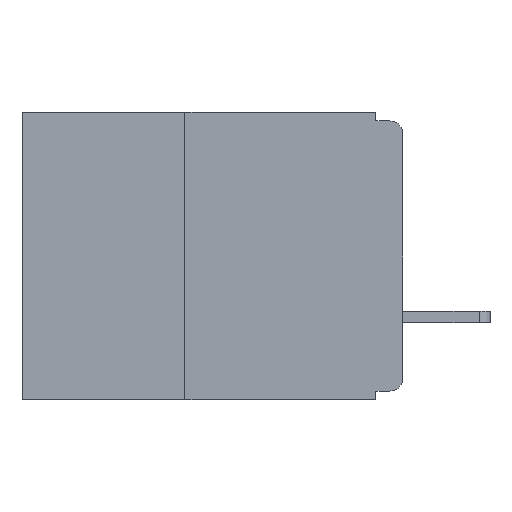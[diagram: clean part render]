
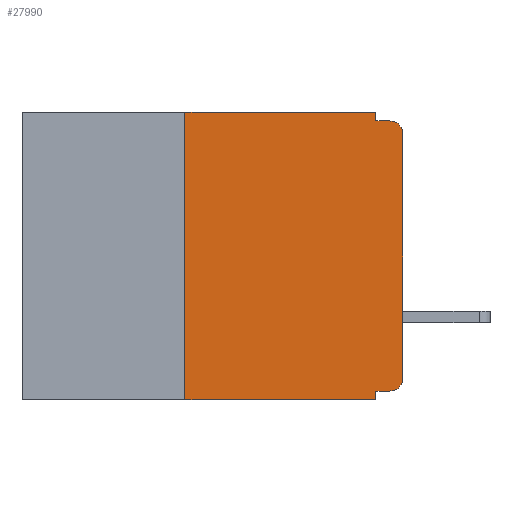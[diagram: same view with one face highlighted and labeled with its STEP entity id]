
A CAD part, left-side view. The second image highlights one B-rep face of the part: STEP entity #27990.
In plain terms, the highlighted planar face has unit normal (-1, 0, 0).
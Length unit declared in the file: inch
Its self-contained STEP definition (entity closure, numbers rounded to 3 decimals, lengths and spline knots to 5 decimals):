
#1207 = DIRECTION ( 'NONE',  ( 0., 0., -1. ) ) ;
#1368 = CARTESIAN_POINT ( 'NONE',  ( 0., 0.015, -0.025 ) ) ;
#1694 = CARTESIAN_POINT ( 'NONE',  ( 0., 0.25, 0. ) ) ;
#2203 = LINE ( 'NONE', #14770, #26049 ) ;
#2496 = ORIENTED_EDGE ( 'NONE', *, *, #6221, .T. ) ;
#2530 = CARTESIAN_POINT ( 'NONE',  ( 0., 0.25, -0.33 ) ) ;
#3075 = DIRECTION ( 'NONE',  ( 0., 1., 0. ) ) ;
#3128 = VERTEX_POINT ( 'NONE', #2530 ) ;
#3298 = VECTOR ( 'NONE', #1207, 39.37008 ) ;
#3785 = DIRECTION ( 'NONE',  ( 0., 0., -1. ) ) ;
#4004 = VERTEX_POINT ( 'NONE', #5722 ) ;
#4083 = CARTESIAN_POINT ( 'NONE',  ( 0., 0.031, 0. ) ) ;
#4739 = CIRCLE ( 'NONE', #28371, 0.015 ) ;
#4760 = PLANE ( 'NONE',  #30239 ) ;
#4867 = DIRECTION ( 'NONE',  ( 1., 0., 0. ) ) ;
#5323 = EDGE_CURVE ( 'NONE', #3128, #28312, #26591, .T. ) ;
#5722 = CARTESIAN_POINT ( 'NONE',  ( 0., 0.015, -0.01 ) ) ;
#6221 = EDGE_CURVE ( 'NONE', #8748, #29144, #20275, .T. ) ;
#6688 = ORIENTED_EDGE ( 'NONE', *, *, #28150, .F. ) ;
#8076 = CARTESIAN_POINT ( 'NONE',  ( 0., 0.437, 0. ) ) ;
#8748 = VERTEX_POINT ( 'NONE', #9443 ) ;
#9213 = EDGE_CURVE ( 'NONE', #29144, #11640, #28932, .T. ) ;
#9443 = CARTESIAN_POINT ( 'NONE',  ( 0., 0.015, -0.32 ) ) ;
#9697 = LINE ( 'NONE', #22633, #3298 ) ;
#9927 = CARTESIAN_POINT ( 'NONE',  ( 0., 0., -0.01 ) ) ;
#10072 = VECTOR ( 'NONE', #18560, 39.37008 ) ;
#10336 = LINE ( 'NONE', #17360, #21491 ) ;
#10445 = ORIENTED_EDGE ( 'NONE', *, *, #21744, .T. ) ;
#10492 = DIRECTION ( 'NONE',  ( 0., -1., 0. ) ) ;
#10761 = EDGE_CURVE ( 'NONE', #30375, #4004, #23723, .T. ) ;
#10952 = CARTESIAN_POINT ( 'NONE',  ( 0., 0.031, -0.33 ) ) ;
#11640 = VERTEX_POINT ( 'NONE', #15917 ) ;
#13031 = ORIENTED_EDGE ( 'NONE', *, *, #10761, .F. ) ;
#13276 = FACE_OUTER_BOUND ( 'NONE', #29593, .T. ) ;
#13622 = LINE ( 'NONE', #8076, #26221 ) ;
#14532 = ORIENTED_EDGE ( 'NONE', *, *, #20973, .F. ) ;
#14658 = CARTESIAN_POINT ( 'NONE',  ( 0., 0., -0.305 ) ) ;
#14770 = CARTESIAN_POINT ( 'NONE',  ( 0., 0.031, -0.33 ) ) ;
#14915 = EDGE_CURVE ( 'NONE', #3128, #23696, #10336, .T. ) ;
#15134 = VERTEX_POINT ( 'NONE', #4083 ) ;
#15917 = CARTESIAN_POINT ( 'NONE',  ( 0., 0., -0.025 ) ) ;
#16177 = CARTESIAN_POINT ( 'NONE',  ( 0., 0., 0. ) ) ;
#16654 = VECTOR ( 'NONE', #28846, 39.37008 ) ;
#17019 = ORIENTED_EDGE ( 'NONE', *, *, #20787, .F. ) ;
#17360 = CARTESIAN_POINT ( 'NONE',  ( 0., 0.25, -0.33 ) ) ;
#17471 = DIRECTION ( 'NONE',  ( 0., 0., -1. ) ) ;
#17504 = DIRECTION ( 'NONE',  ( -1., 0., 0. ) ) ;
#17512 = EDGE_CURVE ( 'NONE', #23696, #15134, #13622, .T. ) ;
#17547 = CARTESIAN_POINT ( 'NONE',  ( 0., 0.015, -0.305 ) ) ;
#18110 = DIRECTION ( 'NONE',  ( -1., 0., 0. ) ) ;
#18560 = DIRECTION ( 'NONE',  ( 0., 0., 1. ) ) ;
#19185 = CARTESIAN_POINT ( 'NONE',  ( 0., 0.437, 0. ) ) ;
#19574 = ORIENTED_EDGE ( 'NONE', *, *, #14915, .F. ) ;
#20079 = VERTEX_POINT ( 'NONE', #26291 ) ;
#20275 = CIRCLE ( 'NONE', #23459, 0.015 ) ;
#20713 = VECTOR ( 'NONE', #3075, 39.37008 ) ;
#20787 = EDGE_CURVE ( 'NONE', #20079, #28312, #2203, .T. ) ;
#20973 = EDGE_CURVE ( 'NONE', #15134, #30375, #9697, .T. ) ;
#21491 = VECTOR ( 'NONE', #24645, 39.37008 ) ;
#21572 = DIRECTION ( 'NONE',  ( 0., 0., -1. ) ) ;
#21744 = EDGE_CURVE ( 'NONE', #11640, #4004, #4739, .T. ) ;
#21856 = ORIENTED_EDGE ( 'NONE', *, *, #5323, .T. ) ;
#22633 = CARTESIAN_POINT ( 'NONE',  ( 0., 0.031, 0. ) ) ;
#22808 = ORIENTED_EDGE ( 'NONE', *, *, #17512, .F. ) ;
#23339 = CARTESIAN_POINT ( 'NONE',  ( 0., 0.031, -0.01 ) ) ;
#23459 = AXIS2_PLACEMENT_3D ( 'NONE', #17547, #17504, #17471 ) ;
#23696 = VERTEX_POINT ( 'NONE', #1694 ) ;
#23723 = LINE ( 'NONE', #9927, #16654 ) ;
#24450 = CARTESIAN_POINT ( 'NONE',  ( 0., 0., -0.32 ) ) ;
#24645 = DIRECTION ( 'NONE',  ( 0., 0., 1. ) ) ;
#25876 = VECTOR ( 'NONE', #30427, 39.37008 ) ;
#26049 = VECTOR ( 'NONE', #26643, 39.37008 ) ;
#26221 = VECTOR ( 'NONE', #10492, 39.37008 ) ;
#26291 = CARTESIAN_POINT ( 'NONE',  ( 0., 0.031, -0.32 ) ) ;
#26591 = LINE ( 'NONE', #29285, #25876 ) ;
#26643 = DIRECTION ( 'NONE',  ( 0., 0., -1. ) ) ;
#26955 = LINE ( 'NONE', #24450, #20713 ) ;
#27990 = ADVANCED_FACE ( 'NONE', ( #13276 ), #4760, .F. ) ;
#28030 = ORIENTED_EDGE ( 'NONE', *, *, #9213, .T. ) ;
#28150 = EDGE_CURVE ( 'NONE', #8748, #20079, #26955, .T. ) ;
#28312 = VERTEX_POINT ( 'NONE', #10952 ) ;
#28371 = AXIS2_PLACEMENT_3D ( 'NONE', #1368, #18110, #3785 ) ;
#28846 = DIRECTION ( 'NONE',  ( 0., -1., 0. ) ) ;
#28932 = LINE ( 'NONE', #16177, #10072 ) ;
#29144 = VERTEX_POINT ( 'NONE', #14658 ) ;
#29285 = CARTESIAN_POINT ( 'NONE',  ( 0., 0.437, -0.33 ) ) ;
#29593 = EDGE_LOOP ( 'NONE', ( #28030, #10445, #13031, #14532, #22808, #19574, #21856, #17019, #6688, #2496 ) ) ;
#30239 = AXIS2_PLACEMENT_3D ( 'NONE', #19185, #4867, #21572 ) ;
#30375 = VERTEX_POINT ( 'NONE', #23339 ) ;
#30427 = DIRECTION ( 'NONE',  ( 0., -1., 0. ) ) ;
